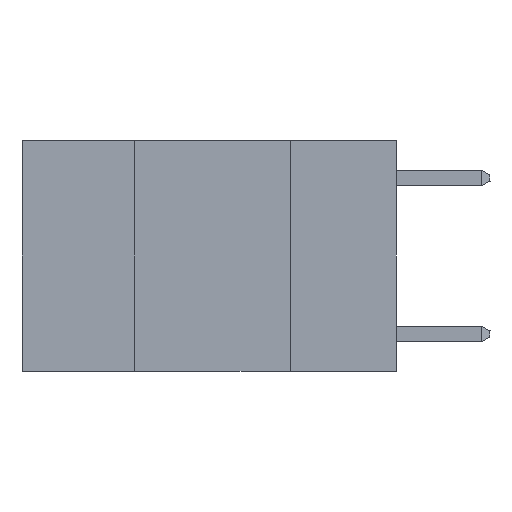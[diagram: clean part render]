
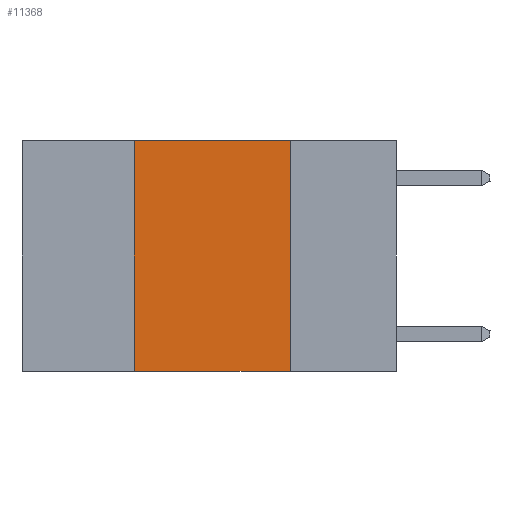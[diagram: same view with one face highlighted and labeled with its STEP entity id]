
A CAD part, left-side view. The second image highlights one B-rep face of the part: STEP entity #11368.
In plain terms, the highlighted planar face has unit normal (-1, 0, 0).
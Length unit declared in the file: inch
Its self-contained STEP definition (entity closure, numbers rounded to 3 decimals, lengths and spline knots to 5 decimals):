
#1365 = LINE ( 'NONE', #18971, #25751 ) ;
#1706 = VECTOR ( 'NONE', #23312, 39.37008 ) ;
#2668 = VERTEX_POINT ( 'NONE', #8233 ) ;
#4164 = DIRECTION ( 'NONE',  ( 0., 0., -1. ) ) ;
#5056 = EDGE_CURVE ( 'NONE', #2668, #26528, #1365, .T. ) ;
#7636 = ORIENTED_EDGE ( 'NONE', *, *, #14899, .F. ) ;
#8233 = CARTESIAN_POINT ( 'NONE',  ( 0., 0.42, 0. ) ) ;
#8411 = CARTESIAN_POINT ( 'NONE',  ( 0., 0.42, 0. ) ) ;
#9704 = AXIS2_PLACEMENT_3D ( 'NONE', #15877, #22521, #13863 ) ;
#10065 = LINE ( 'NONE', #27624, #25052 ) ;
#10650 = CARTESIAN_POINT ( 'NONE',  ( 0., 0.17, -0.37 ) ) ;
#10698 = LINE ( 'NONE', #17089, #19225 ) ;
#11368 = ADVANCED_FACE ( 'NONE', ( #15077 ), #17058, .F. ) ;
#12339 = CARTESIAN_POINT ( 'NONE',  ( 0., 0.42, -0.37 ) ) ;
#13356 = ORIENTED_EDGE ( 'NONE', *, *, #5056, .F. ) ;
#13863 = DIRECTION ( 'NONE',  ( 0., 0., -1. ) ) ;
#14171 = VERTEX_POINT ( 'NONE', #12339 ) ;
#14814 = LINE ( 'NONE', #8411, #1706 ) ;
#14899 = EDGE_CURVE ( 'NONE', #26528, #21665, #10698, .T. ) ;
#15077 = FACE_OUTER_BOUND ( 'NONE', #24233, .T. ) ;
#15877 = CARTESIAN_POINT ( 'NONE',  ( 0., 0.6, 0. ) ) ;
#16567 = DIRECTION ( 'NONE',  ( 0., -1., 0. ) ) ;
#17058 = PLANE ( 'NONE',  #9704 ) ;
#17089 = CARTESIAN_POINT ( 'NONE',  ( 0., 0.17, 0. ) ) ;
#18727 = DIRECTION ( 'NONE',  ( 0., -1., 0. ) ) ;
#18971 = CARTESIAN_POINT ( 'NONE',  ( 0., 0.6, 0. ) ) ;
#19225 = VECTOR ( 'NONE', #4164, 39.37008 ) ;
#20268 = ORIENTED_EDGE ( 'NONE', *, *, #21270, .F. ) ;
#21270 = EDGE_CURVE ( 'NONE', #14171, #2668, #14814, .T. ) ;
#21665 = VERTEX_POINT ( 'NONE', #10650 ) ;
#22083 = ORIENTED_EDGE ( 'NONE', *, *, #26789, .T. ) ;
#22521 = DIRECTION ( 'NONE',  ( 1., 0., 0. ) ) ;
#23312 = DIRECTION ( 'NONE',  ( 0., 0., 1. ) ) ;
#24233 = EDGE_LOOP ( 'NONE', ( #7636, #13356, #20268, #22083 ) ) ;
#25052 = VECTOR ( 'NONE', #18727, 39.37008 ) ;
#25751 = VECTOR ( 'NONE', #16567, 39.37008 ) ;
#26218 = CARTESIAN_POINT ( 'NONE',  ( 0., 0.17, 0. ) ) ;
#26528 = VERTEX_POINT ( 'NONE', #26218 ) ;
#26789 = EDGE_CURVE ( 'NONE', #14171, #21665, #10065, .T. ) ;
#27624 = CARTESIAN_POINT ( 'NONE',  ( 0., 0.6, -0.37 ) ) ;
